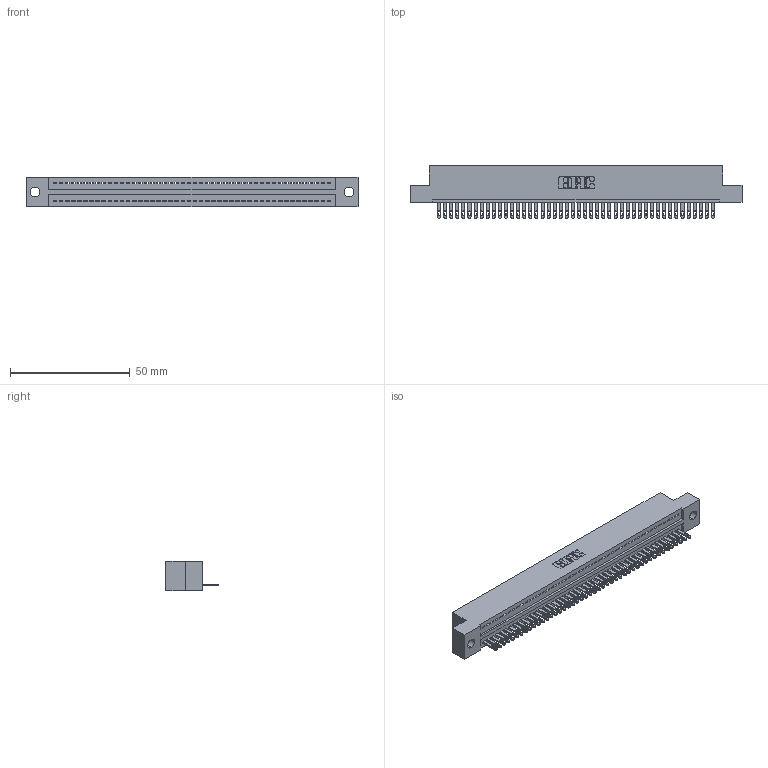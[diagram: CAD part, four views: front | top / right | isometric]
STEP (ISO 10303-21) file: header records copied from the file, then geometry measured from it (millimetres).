
FILE_DESCRIPTION (( 'STEP AP203' ), '1' );
FILE_NAME ('325-046-500-109.STEP', '2020-02-24T22:46:48', ( '' ), ( '' ), 'SwSTEP 2.0', 'SolidWorks 2016', '' );
FILE_SCHEMA (( 'CONFIG_CONTROL_DESIGN' ));
Length unit declared in the file: inch
Products named in the file (3): 325-046-500-109; 325-292-001_325-293-100; 325 Part_.160 TH
Assembly tree (47 placements, depth 2):
  325-046-500-109
    325 Part_.160 TH
    325-292-001_325-293-100  x46
Bounding box: 138.56 x 21.84 x 12.45 mm (x, y, z)
Volume: 17419.1 mm3; surface area: 19101.6 mm2
Topology: 47 solids, 47 shells, 2598 faces, 8039 edges, 5358 vertices
Faces by surface type: plane 1726, cylinder 872
Entity records: 27537 total; most frequent: CARTESIAN_POINT 4756, ORIENTED_EDGE 4738, DIRECTION 4005, EDGE_CURVE 2369, LINE 2237, VECTOR 2237, VERTEX_POINT 1578, AXIS2_PLACEMENT_3D 884
